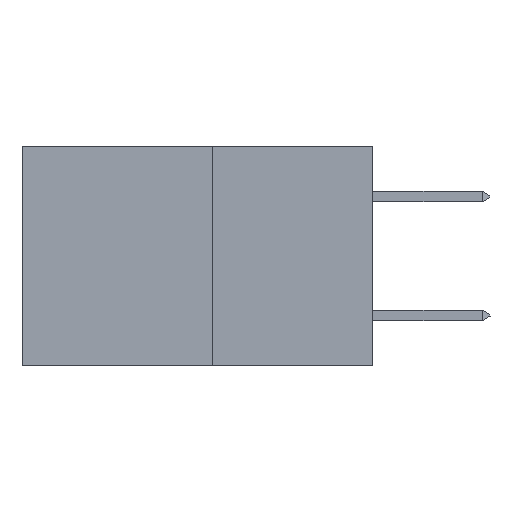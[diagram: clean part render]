
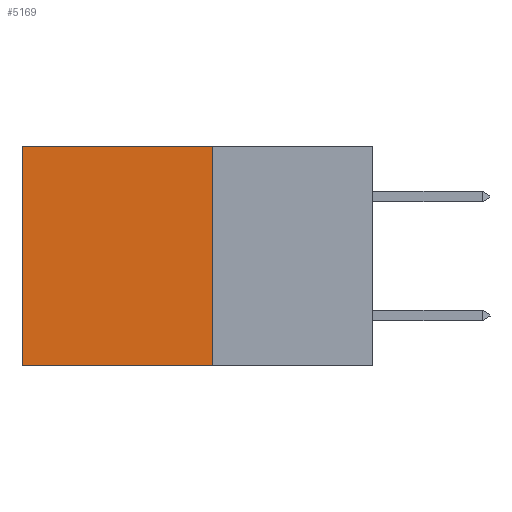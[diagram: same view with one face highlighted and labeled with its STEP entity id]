
A CAD part, left-side view. The second image highlights one B-rep face of the part: STEP entity #5169.
In plain terms, the highlighted planar face has unit normal (-1, 0, 0).
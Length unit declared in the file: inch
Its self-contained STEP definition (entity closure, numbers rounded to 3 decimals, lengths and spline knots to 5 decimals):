
#373 = LINE ( 'NONE', #413, #4245 ) ;
#413 = CARTESIAN_POINT ( 'NONE',  ( 0.277, 0.27, -0.37 ) ) ;
#437 = EDGE_CURVE ( 'NONE', #7828, #6146, #6853, .T. ) ;
#472 = VERTEX_POINT ( 'NONE', #7399 ) ;
#485 = CARTESIAN_POINT ( 'NONE',  ( 0.277, 0.59, -0.37 ) ) ;
#2129 = VECTOR ( 'NONE', #4849, 39.37008 ) ;
#2147 = EDGE_CURVE ( 'NONE', #7828, #472, #8135, .T. ) ;
#2378 = ORIENTED_EDGE ( 'NONE', *, *, #8006, .F. ) ;
#2532 = EDGE_LOOP ( 'NONE', ( #8612, #2378, #9152, #9058 ) ) ;
#2696 = VECTOR ( 'NONE', #4385, 39.37008 ) ;
#2829 = DIRECTION ( 'NONE',  ( 0., 1., 0. ) ) ;
#2984 = VECTOR ( 'NONE', #4862, 39.37008 ) ;
#3223 = AXIS2_PLACEMENT_3D ( 'NONE', #9146, #9392, #7887 ) ;
#4063 = LINE ( 'NONE', #5489, #2129 ) ;
#4245 = VECTOR ( 'NONE', #2829, 39.37008 ) ;
#4385 = DIRECTION ( 'NONE',  ( 0., 0., -1. ) ) ;
#4829 = CARTESIAN_POINT ( 'NONE',  ( 0.277, 0.27, -0.37 ) ) ;
#4849 = DIRECTION ( 'NONE',  ( 0., 0., -1. ) ) ;
#4862 = DIRECTION ( 'NONE',  ( 0., 1., 0. ) ) ;
#5089 = FACE_OUTER_BOUND ( 'NONE', #2532, .T. ) ;
#5169 = ADVANCED_FACE ( 'NONE', ( #5089 ), #6256, .F. ) ;
#5351 = CARTESIAN_POINT ( 'NONE',  ( 0.277, 0.27, 0. ) ) ;
#5489 = CARTESIAN_POINT ( 'NONE',  ( 0.277, 0.59, -0.37 ) ) ;
#5614 = EDGE_CURVE ( 'NONE', #6146, #8799, #4063, .T. ) ;
#5628 = CARTESIAN_POINT ( 'NONE',  ( 0.277, 0.27, 0. ) ) ;
#6146 = VERTEX_POINT ( 'NONE', #8890 ) ;
#6256 = PLANE ( 'NONE',  #3223 ) ;
#6853 = LINE ( 'NONE', #5351, #2984 ) ;
#7399 = CARTESIAN_POINT ( 'NONE',  ( 0.277, 0.27, -0.37 ) ) ;
#7828 = VERTEX_POINT ( 'NONE', #5628 ) ;
#7887 = DIRECTION ( 'NONE',  ( 0., 0., -1. ) ) ;
#8006 = EDGE_CURVE ( 'NONE', #472, #8799, #373, .T. ) ;
#8135 = LINE ( 'NONE', #4829, #2696 ) ;
#8612 = ORIENTED_EDGE ( 'NONE', *, *, #5614, .T. ) ;
#8799 = VERTEX_POINT ( 'NONE', #485 ) ;
#8890 = CARTESIAN_POINT ( 'NONE',  ( 0.277, 0.59, 0. ) ) ;
#9058 = ORIENTED_EDGE ( 'NONE', *, *, #437, .T. ) ;
#9146 = CARTESIAN_POINT ( 'NONE',  ( 0.277, 0.27, -0.37 ) ) ;
#9152 = ORIENTED_EDGE ( 'NONE', *, *, #2147, .F. ) ;
#9392 = DIRECTION ( 'NONE',  ( 1., 0., 0. ) ) ;
